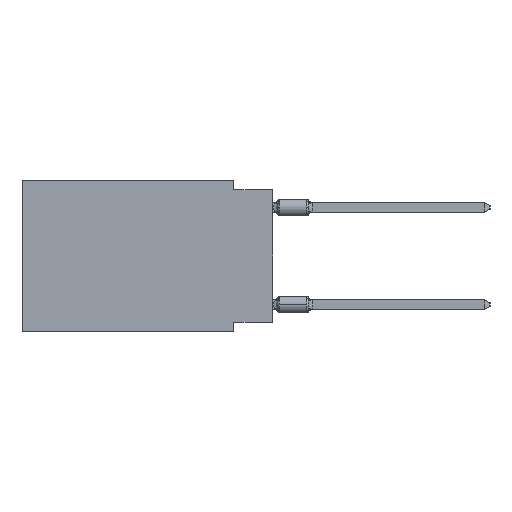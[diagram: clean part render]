
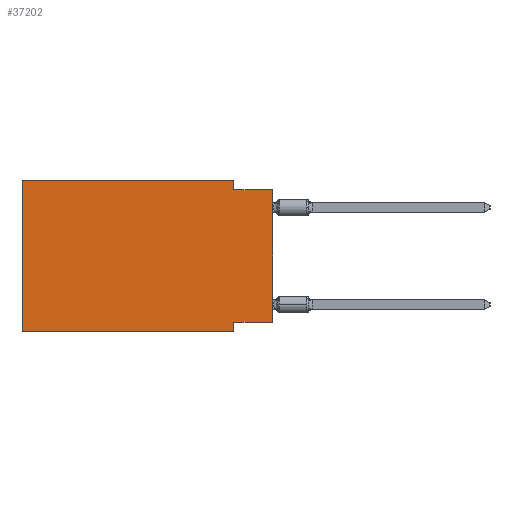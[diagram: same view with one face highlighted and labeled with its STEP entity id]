
A CAD part, left-side view. The second image highlights one B-rep face of the part: STEP entity #37202.
In plain terms, the highlighted planar face has unit normal (-1, 0, 0).
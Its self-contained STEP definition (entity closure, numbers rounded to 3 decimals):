
#33 = VECTOR ( 'NONE', #38575, 1000. ) ;
#494 = CARTESIAN_POINT ( 'NONE',  ( 0., 0., -9.271 ) ) ;
#961 = VECTOR ( 'NONE', #11774, 1000. ) ;
#1712 = LINE ( 'NONE', #20617, #5255 ) ;
#2491 = DIRECTION ( 'NONE',  ( 0., 0., 1. ) ) ;
#3647 = FACE_OUTER_BOUND ( 'NONE', #13273, .T. ) ;
#5255 = VECTOR ( 'NONE', #33257, 1000. ) ;
#7163 = CARTESIAN_POINT ( 'NONE',  ( 0., 16.383, 0. ) ) ;
#7419 = CARTESIAN_POINT ( 'NONE',  ( 0., 16.383, -9.906 ) ) ;
#8200 = LINE ( 'NONE', #20871, #26531 ) ;
#8905 = VECTOR ( 'NONE', #2491, 1000. ) ;
#9130 = CARTESIAN_POINT ( 'NONE',  ( 0., 2.54, 0. ) ) ;
#9488 = VERTEX_POINT ( 'NONE', #20411 ) ;
#9740 = ORIENTED_EDGE ( 'NONE', *, *, #25356, .T. ) ;
#9850 = VECTOR ( 'NONE', #16919, 1000. ) ;
#10070 = DIRECTION ( 'NONE',  ( 1., 0., 0. ) ) ;
#10074 = EDGE_CURVE ( 'NONE', #27463, #30666, #12454, .T. ) ;
#11774 = DIRECTION ( 'NONE',  ( 0., 1., 0. ) ) ;
#12454 = LINE ( 'NONE', #36934, #8905 ) ;
#12764 = VERTEX_POINT ( 'NONE', #30067 ) ;
#12978 = DIRECTION ( 'NONE',  ( 0., 0., -1. ) ) ;
#13273 = EDGE_LOOP ( 'NONE', ( #29310, #16402, #19080, #32858, #29718, #9740, #31815, #20984 ) ) ;
#15001 = CARTESIAN_POINT ( 'NONE',  ( 0., 2.54, 0. ) ) ;
#16402 = ORIENTED_EDGE ( 'NONE', *, *, #20229, .F. ) ;
#16522 = EDGE_CURVE ( 'NONE', #12764, #32815, #39501, .T. ) ;
#16635 = VERTEX_POINT ( 'NONE', #39913 ) ;
#16919 = DIRECTION ( 'NONE',  ( 0., 0., -1. ) ) ;
#17242 = VECTOR ( 'NONE', #22222, 1000. ) ;
#17811 = CARTESIAN_POINT ( 'NONE',  ( 0., 0., -9.271 ) ) ;
#18522 = CARTESIAN_POINT ( 'NONE',  ( 0., 2.54, -9.906 ) ) ;
#19080 = ORIENTED_EDGE ( 'NONE', *, *, #22603, .F. ) ;
#20229 = EDGE_CURVE ( 'NONE', #9488, #30666, #8200, .T. ) ;
#20411 = CARTESIAN_POINT ( 'NONE',  ( 0., 2.54, -0.635 ) ) ;
#20617 = CARTESIAN_POINT ( 'NONE',  ( 0., 16.383, 0. ) ) ;
#20871 = CARTESIAN_POINT ( 'NONE',  ( 0., 0., -0.635 ) ) ;
#20984 = ORIENTED_EDGE ( 'NONE', *, *, #27899, .F. ) ;
#21072 = VERTEX_POINT ( 'NONE', #38209 ) ;
#22222 = DIRECTION ( 'NONE',  ( 0., 0., -1. ) ) ;
#22428 = LINE ( 'NONE', #29254, #33 ) ;
#22603 = EDGE_CURVE ( 'NONE', #35528, #9488, #34241, .T. ) ;
#22739 = EDGE_CURVE ( 'NONE', #16635, #21072, #22428, .T. ) ;
#23737 = AXIS2_PLACEMENT_3D ( 'NONE', #7163, #10070, #12978 ) ;
#25356 = EDGE_CURVE ( 'NONE', #16635, #32815, #40632, .T. ) ;
#26531 = VECTOR ( 'NONE', #34131, 1000. ) ;
#27463 = VERTEX_POINT ( 'NONE', #494 ) ;
#27899 = EDGE_CURVE ( 'NONE', #27463, #12764, #39981, .T. ) ;
#29254 = CARTESIAN_POINT ( 'NONE',  ( 0., 16.383, 0. ) ) ;
#29310 = ORIENTED_EDGE ( 'NONE', *, *, #10074, .T. ) ;
#29718 = ORIENTED_EDGE ( 'NONE', *, *, #22739, .F. ) ;
#30067 = CARTESIAN_POINT ( 'NONE',  ( 0., 2.54, -9.271 ) ) ;
#30666 = VERTEX_POINT ( 'NONE', #39967 ) ;
#31815 = ORIENTED_EDGE ( 'NONE', *, *, #16522, .F. ) ;
#31871 = PLANE ( 'NONE',  #23737 ) ;
#32815 = VERTEX_POINT ( 'NONE', #18522 ) ;
#32858 = ORIENTED_EDGE ( 'NONE', *, *, #33728, .F. ) ;
#33257 = DIRECTION ( 'NONE',  ( 0., -1., 0. ) ) ;
#33728 = EDGE_CURVE ( 'NONE', #21072, #35528, #1712, .T. ) ;
#34131 = DIRECTION ( 'NONE',  ( 0., -1., 0. ) ) ;
#34241 = LINE ( 'NONE', #9130, #17242 ) ;
#35280 = VECTOR ( 'NONE', #38548, 1000. ) ;
#35528 = VERTEX_POINT ( 'NONE', #15001 ) ;
#35600 = CARTESIAN_POINT ( 'NONE',  ( 0., 2.54, -9.906 ) ) ;
#36934 = CARTESIAN_POINT ( 'NONE',  ( 0., 0., 0. ) ) ;
#37202 = ADVANCED_FACE ( 'NONE', ( #3647 ), #31871, .F. ) ;
#38209 = CARTESIAN_POINT ( 'NONE',  ( 0., 16.383, 0. ) ) ;
#38548 = DIRECTION ( 'NONE',  ( 0., -1., 0. ) ) ;
#38575 = DIRECTION ( 'NONE',  ( 0., 0., 1. ) ) ;
#39501 = LINE ( 'NONE', #35600, #9850 ) ;
#39913 = CARTESIAN_POINT ( 'NONE',  ( 0., 16.383, -9.906 ) ) ;
#39967 = CARTESIAN_POINT ( 'NONE',  ( 0., 0., -0.635 ) ) ;
#39981 = LINE ( 'NONE', #17811, #961 ) ;
#40632 = LINE ( 'NONE', #7419, #35280 ) ;
